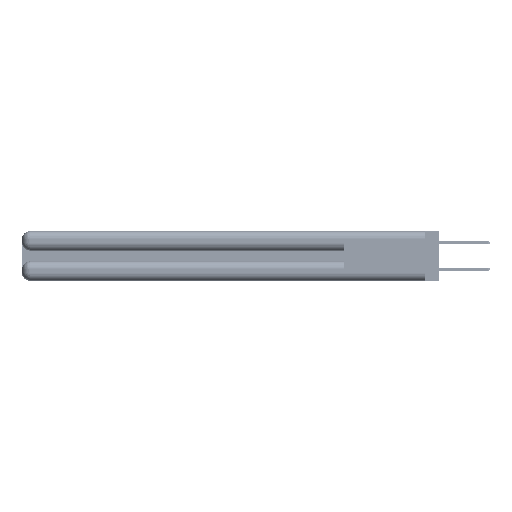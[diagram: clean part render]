
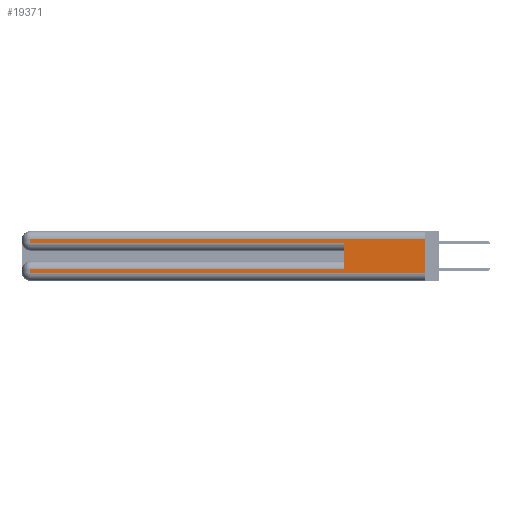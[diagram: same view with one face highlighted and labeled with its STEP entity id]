
A CAD part, left-side view. The second image highlights one B-rep face of the part: STEP entity #19371.
In plain terms, the highlighted planar face has unit normal (-1, 0, 0).
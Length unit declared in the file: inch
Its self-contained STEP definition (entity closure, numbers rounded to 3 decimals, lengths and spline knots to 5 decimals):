
#3256 = EDGE_LOOP ( 'NONE', ( #6105, #4384, #44711, #48568, #24672, #25006, #29178, #25337 ) ) ;
#3267 = DIRECTION ( 'NONE',  ( 0., -1., 0. ) ) ;
#3946 = VECTOR ( 'NONE', #13523, 39.37008 ) ;
#4384 = ORIENTED_EDGE ( 'NONE', *, *, #51868, .T. ) ;
#4897 = LINE ( 'NONE', #24636, #26810 ) ;
#5224 = DIRECTION ( 'NONE',  ( 0., 0., -1. ) ) ;
#5325 = VECTOR ( 'NONE', #23931, 39.37008 ) ;
#6105 = ORIENTED_EDGE ( 'NONE', *, *, #15688, .F. ) ;
#6388 = DIRECTION ( 'NONE',  ( 0., 0., -1. ) ) ;
#10742 = DIRECTION ( 'NONE',  ( 0., 0., -1. ) ) ;
#11007 = CARTESIAN_POINT ( 'NONE',  ( 0., 2.94, 0.085 ) ) ;
#12030 = CARTESIAN_POINT ( 'NONE',  ( 0., 0.6, 0.145 ) ) ;
#13523 = DIRECTION ( 'NONE',  ( 0., 1., 0. ) ) ;
#13859 = EDGE_CURVE ( 'NONE', #32964, #14004, #34857, .T. ) ;
#14004 = VERTEX_POINT ( 'NONE', #38879 ) ;
#14149 = LINE ( 'NONE', #12030, #24398 ) ;
#15211 = VERTEX_POINT ( 'NONE', #25149 ) ;
#15688 = EDGE_CURVE ( 'NONE', #23079, #19180, #40146, .T. ) ;
#15754 = LINE ( 'NONE', #54204, #28777 ) ;
#16221 = DIRECTION ( 'NONE',  ( 0., -1., 0. ) ) ;
#16402 = DIRECTION ( 'NONE',  ( 0., 0., 1. ) ) ;
#19180 = VERTEX_POINT ( 'NONE', #31444 ) ;
#19371 = ADVANCED_FACE ( 'NONE', ( #28170 ), #28193, .F. ) ;
#19394 = CARTESIAN_POINT ( 'NONE',  ( 0., 2.94, 0.06 ) ) ;
#20028 = EDGE_CURVE ( 'NONE', #45558, #41337, #15754, .T. ) ;
#20871 = VECTOR ( 'NONE', #3267, 39.37008 ) ;
#23079 = VERTEX_POINT ( 'NONE', #27931 ) ;
#23931 = DIRECTION ( 'NONE',  ( 0., 0., -1. ) ) ;
#24398 = VECTOR ( 'NONE', #16402, 39.37008 ) ;
#24636 = CARTESIAN_POINT ( 'NONE',  ( 0., 0., 0.085 ) ) ;
#24672 = ORIENTED_EDGE ( 'NONE', *, *, #35387, .F. ) ;
#25006 = ORIENTED_EDGE ( 'NONE', *, *, #42321, .T. ) ;
#25149 = CARTESIAN_POINT ( 'NONE',  ( 0., 0.6, 0.085 ) ) ;
#25337 = ORIENTED_EDGE ( 'NONE', *, *, #50354, .T. ) ;
#26752 = CARTESIAN_POINT ( 'NONE',  ( 0., 2.94, 0.31 ) ) ;
#26773 = CARTESIAN_POINT ( 'NONE',  ( 0., 2.94, 0.285 ) ) ;
#26810 = VECTOR ( 'NONE', #38519, 39.37008 ) ;
#27048 = CARTESIAN_POINT ( 'NONE',  ( 0., 2.94, 0.37 ) ) ;
#27203 = LINE ( 'NONE', #52780, #3946 ) ;
#27931 = CARTESIAN_POINT ( 'NONE',  ( 0., 0., 0.31 ) ) ;
#28170 = FACE_OUTER_BOUND ( 'NONE', #3256, .T. ) ;
#28193 = PLANE ( 'NONE',  #36951 ) ;
#28777 = VECTOR ( 'NONE', #10742, 39.37008 ) ;
#29178 = ORIENTED_EDGE ( 'NONE', *, *, #20028, .T. ) ;
#31444 = CARTESIAN_POINT ( 'NONE',  ( 0., 0., 0.06 ) ) ;
#32127 = VECTOR ( 'NONE', #16221, 39.37008 ) ;
#32564 = DIRECTION ( 'NONE',  ( 1., 0., 0. ) ) ;
#32703 = VECTOR ( 'NONE', #5224, 39.37008 ) ;
#32720 = CARTESIAN_POINT ( 'NONE',  ( 0., 0., 0.37 ) ) ;
#32964 = VERTEX_POINT ( 'NONE', #26773 ) ;
#34318 = EDGE_CURVE ( 'NONE', #44782, #32964, #44266, .T. ) ;
#34857 = LINE ( 'NONE', #37930, #32127 ) ;
#35387 = EDGE_CURVE ( 'NONE', #15211, #14004, #14149, .T. ) ;
#36951 = AXIS2_PLACEMENT_3D ( 'NONE', #49882, #32564, #6388 ) ;
#37930 = CARTESIAN_POINT ( 'NONE',  ( 0., 0., 0.285 ) ) ;
#38519 = DIRECTION ( 'NONE',  ( 0., 1., 0. ) ) ;
#38879 = CARTESIAN_POINT ( 'NONE',  ( 0., 0.6, 0.285 ) ) ;
#40146 = LINE ( 'NONE', #32720, #5325 ) ;
#41337 = VERTEX_POINT ( 'NONE', #19394 ) ;
#42321 = EDGE_CURVE ( 'NONE', #15211, #45558, #4897, .T. ) ;
#44076 = LINE ( 'NONE', #55530, #20871 ) ;
#44266 = LINE ( 'NONE', #27048, #32703 ) ;
#44711 = ORIENTED_EDGE ( 'NONE', *, *, #34318, .T. ) ;
#44782 = VERTEX_POINT ( 'NONE', #26752 ) ;
#45558 = VERTEX_POINT ( 'NONE', #11007 ) ;
#48568 = ORIENTED_EDGE ( 'NONE', *, *, #13859, .T. ) ;
#49882 = CARTESIAN_POINT ( 'NONE',  ( 0., 0., 0.37 ) ) ;
#50354 = EDGE_CURVE ( 'NONE', #41337, #19180, #44076, .T. ) ;
#51868 = EDGE_CURVE ( 'NONE', #23079, #44782, #27203, .T. ) ;
#52780 = CARTESIAN_POINT ( 'NONE',  ( 0., 0., 0.31 ) ) ;
#54204 = CARTESIAN_POINT ( 'NONE',  ( 0., 2.94, 0.37 ) ) ;
#55530 = CARTESIAN_POINT ( 'NONE',  ( 0., 0., 0.06 ) ) ;
